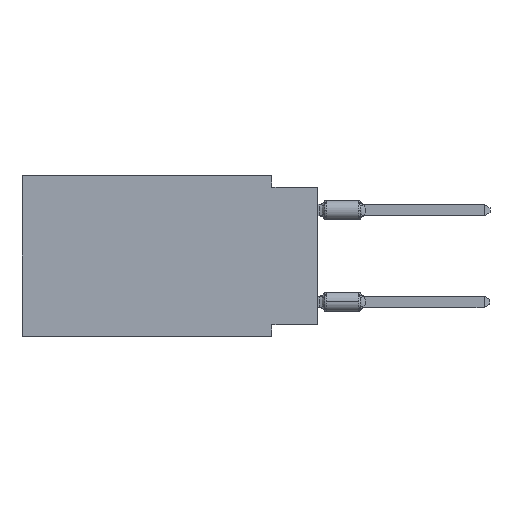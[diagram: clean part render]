
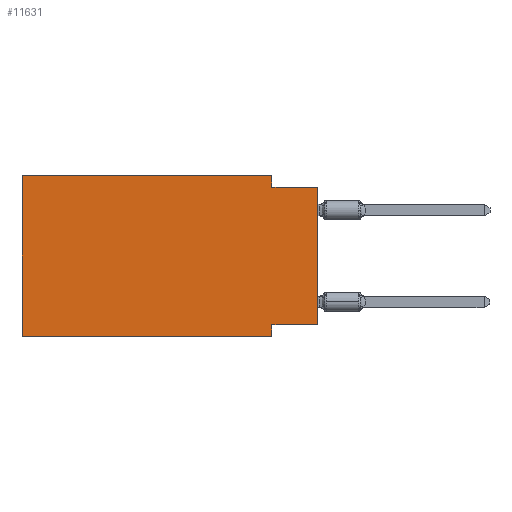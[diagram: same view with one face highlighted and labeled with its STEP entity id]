
A CAD part, left-side view. The second image highlights one B-rep face of the part: STEP entity #11631.
In plain terms, the highlighted planar face has unit normal (-1, 0, 0).
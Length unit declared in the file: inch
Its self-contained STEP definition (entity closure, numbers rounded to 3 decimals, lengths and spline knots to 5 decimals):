
#66 = VECTOR ( 'NONE', #5211, 39.37008 ) ;
#140 = CARTESIAN_POINT ( 'NONE',  ( 0., 0.1, 0. ) ) ;
#364 = CARTESIAN_POINT ( 'NONE',  ( 0., 0.645, 0. ) ) ;
#503 = DIRECTION ( 'NONE',  ( 0., -1., 0. ) ) ;
#971 = VECTOR ( 'NONE', #17464, 39.37008 ) ;
#1131 = EDGE_LOOP ( 'NONE', ( #6246, #17036, #4849, #4978, #10652, #12563, #14182, #2123 ) ) ;
#1287 = LINE ( 'NONE', #5456, #2342 ) ;
#1758 = CARTESIAN_POINT ( 'NONE',  ( 0., 0.645, 0. ) ) ;
#1798 = EDGE_CURVE ( 'NONE', #14269, #13406, #4800, .T. ) ;
#2123 = ORIENTED_EDGE ( 'NONE', *, *, #14902, .F. ) ;
#2203 = VECTOR ( 'NONE', #3862, 39.37008 ) ;
#2342 = VECTOR ( 'NONE', #3881, 39.37008 ) ;
#2517 = VERTEX_POINT ( 'NONE', #6930 ) ;
#3862 = DIRECTION ( 'NONE',  ( 0., 1., 0. ) ) ;
#3881 = DIRECTION ( 'NONE',  ( 0., -1., 0. ) ) ;
#4578 = EDGE_CURVE ( 'NONE', #7716, #2517, #12095, .T. ) ;
#4642 = DIRECTION ( 'NONE',  ( 0., 0., -1. ) ) ;
#4732 = PLANE ( 'NONE',  #13093 ) ;
#4800 = LINE ( 'NONE', #13373, #6660 ) ;
#4849 = ORIENTED_EDGE ( 'NONE', *, *, #4578, .F. ) ;
#4978 = ORIENTED_EDGE ( 'NONE', *, *, #10433, .F. ) ;
#5183 = CARTESIAN_POINT ( 'NONE',  ( 0., 0., -0.025 ) ) ;
#5211 = DIRECTION ( 'NONE',  ( 0., 0., -1. ) ) ;
#5456 = CARTESIAN_POINT ( 'NONE',  ( 0., 0., -0.025 ) ) ;
#5578 = VERTEX_POINT ( 'NONE', #5957 ) ;
#5957 = CARTESIAN_POINT ( 'NONE',  ( 0., 0.1, -0.35 ) ) ;
#6246 = ORIENTED_EDGE ( 'NONE', *, *, #10435, .T. ) ;
#6660 = VECTOR ( 'NONE', #12975, 39.37008 ) ;
#6717 = EDGE_CURVE ( 'NONE', #14269, #5578, #14649, .T. ) ;
#6834 = CARTESIAN_POINT ( 'NONE',  ( 0., 0., -0.325 ) ) ;
#6930 = CARTESIAN_POINT ( 'NONE',  ( 0., 0.1, -0.025 ) ) ;
#7244 = EDGE_CURVE ( 'NONE', #9989, #5578, #17955, .T. ) ;
#7410 = DIRECTION ( 'NONE',  ( 0., -1., 0. ) ) ;
#7554 = CARTESIAN_POINT ( 'NONE',  ( 0., 0.645, -0.35 ) ) ;
#7716 = VERTEX_POINT ( 'NONE', #140 ) ;
#8495 = CARTESIAN_POINT ( 'NONE',  ( 0., 0., -0.325 ) ) ;
#8651 = VECTOR ( 'NONE', #503, 39.37008 ) ;
#9989 = VERTEX_POINT ( 'NONE', #11821 ) ;
#10205 = LINE ( 'NONE', #1758, #15809 ) ;
#10243 = DIRECTION ( 'NONE',  ( 0., 0., -1. ) ) ;
#10433 = EDGE_CURVE ( 'NONE', #13406, #7716, #10205, .T. ) ;
#10435 = EDGE_CURVE ( 'NONE', #17105, #11647, #15694, .T. ) ;
#10652 = ORIENTED_EDGE ( 'NONE', *, *, #1798, .F. ) ;
#11631 = ADVANCED_FACE ( 'NONE', ( #13092 ), #4732, .F. ) ;
#11647 = VERTEX_POINT ( 'NONE', #5183 ) ;
#11698 = DIRECTION ( 'NONE',  ( 1., 0., 0. ) ) ;
#11821 = CARTESIAN_POINT ( 'NONE',  ( 0., 0.1, -0.325 ) ) ;
#12073 = CARTESIAN_POINT ( 'NONE',  ( 0., 0.645, -0.35 ) ) ;
#12095 = LINE ( 'NONE', #13328, #13101 ) ;
#12563 = ORIENTED_EDGE ( 'NONE', *, *, #6717, .T. ) ;
#12975 = DIRECTION ( 'NONE',  ( 0., 0., 1. ) ) ;
#13088 = CARTESIAN_POINT ( 'NONE',  ( 0., 0., 0. ) ) ;
#13092 = FACE_OUTER_BOUND ( 'NONE', #1131, .T. ) ;
#13093 = AXIS2_PLACEMENT_3D ( 'NONE', #364, #11698, #4642 ) ;
#13101 = VECTOR ( 'NONE', #10243, 39.37008 ) ;
#13328 = CARTESIAN_POINT ( 'NONE',  ( 0., 0.1, 0. ) ) ;
#13373 = CARTESIAN_POINT ( 'NONE',  ( 0., 0.645, 0. ) ) ;
#13406 = VERTEX_POINT ( 'NONE', #14712 ) ;
#14182 = ORIENTED_EDGE ( 'NONE', *, *, #7244, .F. ) ;
#14269 = VERTEX_POINT ( 'NONE', #12073 ) ;
#14649 = LINE ( 'NONE', #7554, #8651 ) ;
#14712 = CARTESIAN_POINT ( 'NONE',  ( 0., 0.645, 0. ) ) ;
#14902 = EDGE_CURVE ( 'NONE', #17105, #9989, #15299, .T. ) ;
#15299 = LINE ( 'NONE', #8495, #2203 ) ;
#15694 = LINE ( 'NONE', #13088, #971 ) ;
#15809 = VECTOR ( 'NONE', #7410, 39.37008 ) ;
#16208 = CARTESIAN_POINT ( 'NONE',  ( 0., 0.1, -0.35 ) ) ;
#17011 = EDGE_CURVE ( 'NONE', #2517, #11647, #1287, .T. ) ;
#17036 = ORIENTED_EDGE ( 'NONE', *, *, #17011, .F. ) ;
#17105 = VERTEX_POINT ( 'NONE', #6834 ) ;
#17464 = DIRECTION ( 'NONE',  ( 0., 0., 1. ) ) ;
#17955 = LINE ( 'NONE', #16208, #66 ) ;
